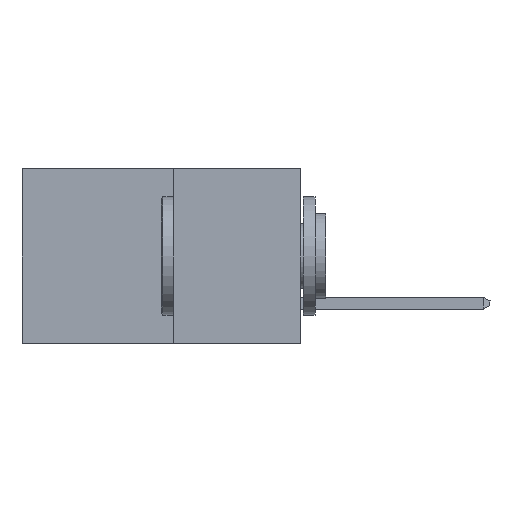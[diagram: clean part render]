
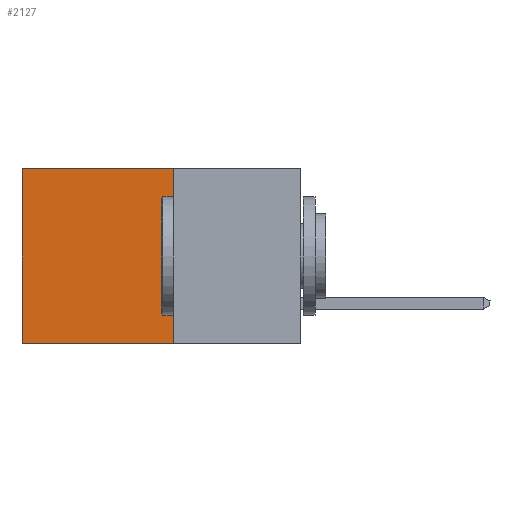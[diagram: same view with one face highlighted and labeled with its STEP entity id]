
A CAD part, left-side view. The second image highlights one B-rep face of the part: STEP entity #2127.
In plain terms, the highlighted planar face has unit normal (-1, 0, 0).
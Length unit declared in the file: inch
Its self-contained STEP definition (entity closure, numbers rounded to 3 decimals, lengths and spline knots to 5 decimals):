
#1235 = VECTOR ( 'NONE', #5435, 39.37008 ) ;
#1625 = CARTESIAN_POINT ( 'NONE',  ( 0.277, 0.27, 0. ) ) ;
#2127 = ADVANCED_FACE ( 'NONE', ( #18147 ), #15046, .F. ) ;
#3064 = EDGE_LOOP ( 'NONE', ( #5672, #23629, #12177, #9514 ) ) ;
#3499 = DIRECTION ( 'NONE',  ( 0., 1., 0. ) ) ;
#5435 = DIRECTION ( 'NONE',  ( 0., 0., -1. ) ) ;
#5445 = DIRECTION ( 'NONE',  ( 0., 0., -1. ) ) ;
#5672 = ORIENTED_EDGE ( 'NONE', *, *, #15667, .T. ) ;
#5966 = VECTOR ( 'NONE', #3499, 39.37008 ) ;
#6548 = LINE ( 'NONE', #16914, #5966 ) ;
#7924 = VECTOR ( 'NONE', #17266, 39.37008 ) ;
#8659 = LINE ( 'NONE', #11080, #12016 ) ;
#9514 = ORIENTED_EDGE ( 'NONE', *, *, #13744, .T. ) ;
#10006 = CARTESIAN_POINT ( 'NONE',  ( 0.277, 0.59, 0. ) ) ;
#10512 = EDGE_CURVE ( 'NONE', #24550, #10741, #21591, .T. ) ;
#10570 = VERTEX_POINT ( 'NONE', #20816 ) ;
#10741 = VERTEX_POINT ( 'NONE', #13754 ) ;
#11080 = CARTESIAN_POINT ( 'NONE',  ( 0.277, 0.59, -0.37 ) ) ;
#12016 = VECTOR ( 'NONE', #5445, 39.37008 ) ;
#12088 = VERTEX_POINT ( 'NONE', #10006 ) ;
#12177 = ORIENTED_EDGE ( 'NONE', *, *, #10512, .F. ) ;
#13744 = EDGE_CURVE ( 'NONE', #24550, #12088, #6548, .T. ) ;
#13754 = CARTESIAN_POINT ( 'NONE',  ( 0.277, 0.27, -0.37 ) ) ;
#14225 = LINE ( 'NONE', #15393, #7924 ) ;
#14554 = AXIS2_PLACEMENT_3D ( 'NONE', #16961, #18457, #18537 ) ;
#14983 = CARTESIAN_POINT ( 'NONE',  ( 0.277, 0.27, -0.37 ) ) ;
#15046 = PLANE ( 'NONE',  #14554 ) ;
#15393 = CARTESIAN_POINT ( 'NONE',  ( 0.277, 0.27, -0.37 ) ) ;
#15667 = EDGE_CURVE ( 'NONE', #12088, #10570, #8659, .T. ) ;
#16914 = CARTESIAN_POINT ( 'NONE',  ( 0.277, 0.27, 0. ) ) ;
#16961 = CARTESIAN_POINT ( 'NONE',  ( 0.277, 0.27, -0.37 ) ) ;
#17266 = DIRECTION ( 'NONE',  ( 0., 1., 0. ) ) ;
#18147 = FACE_OUTER_BOUND ( 'NONE', #3064, .T. ) ;
#18457 = DIRECTION ( 'NONE',  ( 1., 0., 0. ) ) ;
#18537 = DIRECTION ( 'NONE',  ( 0., 0., -1. ) ) ;
#20816 = CARTESIAN_POINT ( 'NONE',  ( 0.277, 0.59, -0.37 ) ) ;
#21541 = EDGE_CURVE ( 'NONE', #10741, #10570, #14225, .T. ) ;
#21591 = LINE ( 'NONE', #14983, #1235 ) ;
#23629 = ORIENTED_EDGE ( 'NONE', *, *, #21541, .F. ) ;
#24550 = VERTEX_POINT ( 'NONE', #1625 ) ;
